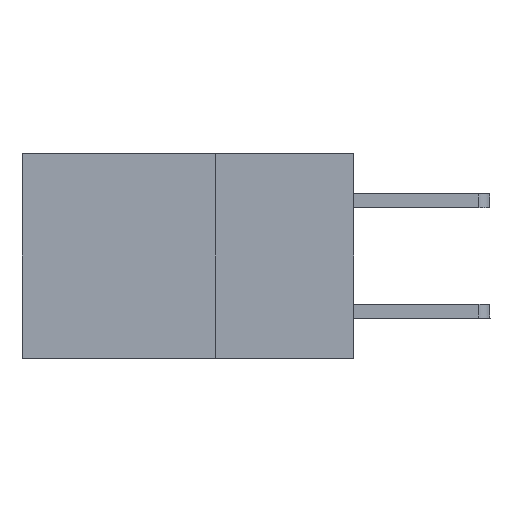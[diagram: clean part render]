
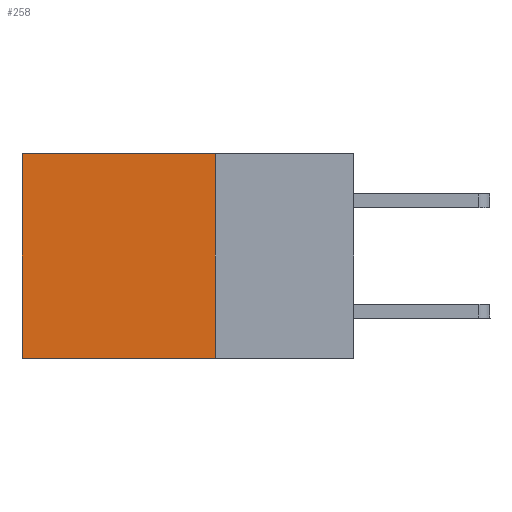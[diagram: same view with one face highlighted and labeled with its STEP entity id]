
A CAD part, left-side view. The second image highlights one B-rep face of the part: STEP entity #258.
In plain terms, the highlighted planar face has unit normal (-1, 0, 0).
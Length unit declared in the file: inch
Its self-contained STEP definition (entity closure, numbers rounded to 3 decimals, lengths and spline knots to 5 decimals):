
#111 = CARTESIAN_POINT ( 'NONE',  ( 0.2875, 0.25, 0. ) ) ;
#258 = ADVANCED_FACE ( 'NONE', ( #2364 ), #2190, .F. ) ;
#471 = DIRECTION ( 'NONE',  ( 0., 0., -1. ) ) ;
#491 = ORIENTED_EDGE ( 'NONE', *, *, #1490, .T. ) ;
#1490 = EDGE_CURVE ( 'NONE', #6105, #2454, #11084, .T. ) ;
#2005 = VECTOR ( 'NONE', #5676, 39.37008 ) ;
#2071 = DIRECTION ( 'NONE',  ( 1., 0., 0. ) ) ;
#2190 = PLANE ( 'NONE',  #5188 ) ;
#2364 = FACE_OUTER_BOUND ( 'NONE', #4305, .T. ) ;
#2376 = VECTOR ( 'NONE', #6644, 39.37008 ) ;
#2454 = VERTEX_POINT ( 'NONE', #2643 ) ;
#2643 = CARTESIAN_POINT ( 'NONE',  ( 0.2875, 0.6, -0.37 ) ) ;
#2961 = CARTESIAN_POINT ( 'NONE',  ( 0.2875, 0.25, -0.37 ) ) ;
#3335 = DIRECTION ( 'NONE',  ( 0., 1., 0. ) ) ;
#4305 = EDGE_LOOP ( 'NONE', ( #491, #7376, #7033, #8100 ) ) ;
#4532 = LINE ( 'NONE', #6101, #11161 ) ;
#4721 = VECTOR ( 'NONE', #8972, 39.37008 ) ;
#4892 = CARTESIAN_POINT ( 'NONE',  ( 0.2875, 0.6, 0. ) ) ;
#5188 = AXIS2_PLACEMENT_3D ( 'NONE', #111, #2071, #471 ) ;
#5241 = CARTESIAN_POINT ( 'NONE',  ( 0.2875, 0.6, 0. ) ) ;
#5676 = DIRECTION ( 'NONE',  ( 0., 0., -1. ) ) ;
#6101 = CARTESIAN_POINT ( 'NONE',  ( 0.2875, 0.25, 0. ) ) ;
#6105 = VERTEX_POINT ( 'NONE', #5241 ) ;
#6644 = DIRECTION ( 'NONE',  ( 0., 1., 0. ) ) ;
#6825 = LINE ( 'NONE', #9184, #2005 ) ;
#7033 = ORIENTED_EDGE ( 'NONE', *, *, #9867, .F. ) ;
#7376 = ORIENTED_EDGE ( 'NONE', *, *, #9214, .F. ) ;
#7533 = VERTEX_POINT ( 'NONE', #9734 ) ;
#8100 = ORIENTED_EDGE ( 'NONE', *, *, #11221, .T. ) ;
#8972 = DIRECTION ( 'NONE',  ( 0., 0., -1. ) ) ;
#9184 = CARTESIAN_POINT ( 'NONE',  ( 0.2875, 0.25, 0. ) ) ;
#9214 = EDGE_CURVE ( 'NONE', #7533, #2454, #9220, .T. ) ;
#9220 = LINE ( 'NONE', #2961, #2376 ) ;
#9239 = VERTEX_POINT ( 'NONE', #10074 ) ;
#9734 = CARTESIAN_POINT ( 'NONE',  ( 0.2875, 0.25, -0.37 ) ) ;
#9867 = EDGE_CURVE ( 'NONE', #9239, #7533, #6825, .T. ) ;
#10074 = CARTESIAN_POINT ( 'NONE',  ( 0.2875, 0.25, 0. ) ) ;
#11084 = LINE ( 'NONE', #4892, #4721 ) ;
#11161 = VECTOR ( 'NONE', #3335, 39.37008 ) ;
#11221 = EDGE_CURVE ( 'NONE', #9239, #6105, #4532, .T. ) ;
